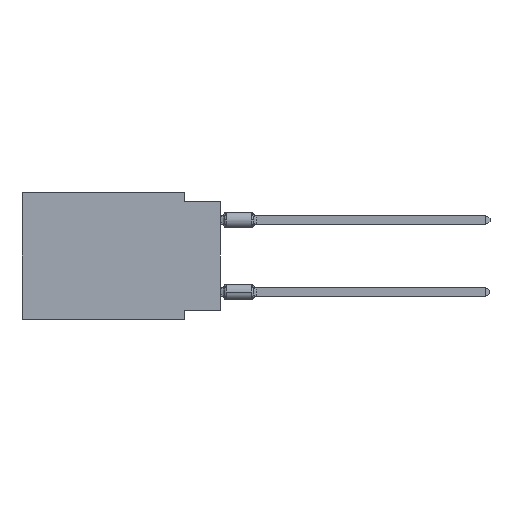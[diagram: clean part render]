
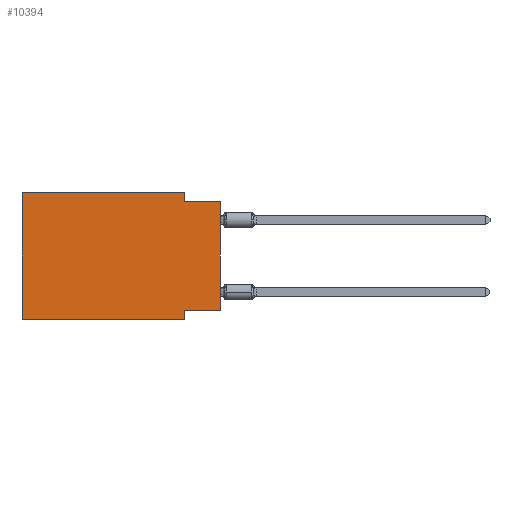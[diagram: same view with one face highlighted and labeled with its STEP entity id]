
A CAD part, left-side view. The second image highlights one B-rep face of the part: STEP entity #10394.
In plain terms, the highlighted planar face has unit normal (-1, 0, 0).
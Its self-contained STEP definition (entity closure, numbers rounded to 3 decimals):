
#94 = EDGE_CURVE ( 'NONE', #20671, #5202, #18886, .T. ) ;
#200 = LINE ( 'NONE', #1727, #14574 ) ;
#619 = CARTESIAN_POINT ( 'NONE',  ( 0., 13.97, -8.89 ) ) ;
#1194 = CARTESIAN_POINT ( 'NONE',  ( 0., 0., -0.635 ) ) ;
#1363 = ORIENTED_EDGE ( 'NONE', *, *, #13516, .F. ) ;
#1425 = PLANE ( 'NONE',  #19031 ) ;
#1727 = CARTESIAN_POINT ( 'NONE',  ( 0., 13.97, 0. ) ) ;
#1982 = EDGE_CURVE ( 'NONE', #8667, #16884, #11767, .T. ) ;
#2257 = CARTESIAN_POINT ( 'NONE',  ( 0., 2.54, -8.89 ) ) ;
#2622 = DIRECTION ( 'NONE',  ( 0., 0., 1. ) ) ;
#2673 = CARTESIAN_POINT ( 'NONE',  ( 0., 13.97, -8.89 ) ) ;
#2741 = EDGE_CURVE ( 'NONE', #5413, #16008, #200, .T. ) ;
#3243 = VERTEX_POINT ( 'NONE', #19959 ) ;
#3809 = VECTOR ( 'NONE', #13233, 1000. ) ;
#4658 = LINE ( 'NONE', #11383, #3809 ) ;
#4990 = VECTOR ( 'NONE', #8406, 1000. ) ;
#5202 = VERTEX_POINT ( 'NONE', #10467 ) ;
#5413 = VERTEX_POINT ( 'NONE', #13486 ) ;
#5815 = CARTESIAN_POINT ( 'NONE',  ( 0., 2.54, -0.635 ) ) ;
#6433 = FACE_OUTER_BOUND ( 'NONE', #13470, .T. ) ;
#6672 = DIRECTION ( 'NONE',  ( 0., 0., 1. ) ) ;
#6986 = LINE ( 'NONE', #8720, #14095 ) ;
#7366 = LINE ( 'NONE', #2257, #20247 ) ;
#7797 = CARTESIAN_POINT ( 'NONE',  ( 0., 2.54, 0. ) ) ;
#8099 = EDGE_CURVE ( 'NONE', #17785, #5202, #7366, .T. ) ;
#8141 = ORIENTED_EDGE ( 'NONE', *, *, #1982, .F. ) ;
#8174 = CARTESIAN_POINT ( 'NONE',  ( 0., 13.97, 0. ) ) ;
#8406 = DIRECTION ( 'NONE',  ( 0., -1., 0. ) ) ;
#8667 = VERTEX_POINT ( 'NONE', #5815 ) ;
#8720 = CARTESIAN_POINT ( 'NONE',  ( 0., 13.97, 0. ) ) ;
#8890 = DIRECTION ( 'NONE',  ( 0., 0., -1. ) ) ;
#9154 = ORIENTED_EDGE ( 'NONE', *, *, #8099, .F. ) ;
#9872 = VECTOR ( 'NONE', #15919, 1000. ) ;
#9995 = ORIENTED_EDGE ( 'NONE', *, *, #2741, .F. ) ;
#10394 = ADVANCED_FACE ( 'NONE', ( #6433 ), #1425, .F. ) ;
#10467 = CARTESIAN_POINT ( 'NONE',  ( 0., 2.54, -8.89 ) ) ;
#11089 = CARTESIAN_POINT ( 'NONE',  ( 0., 0., 0. ) ) ;
#11383 = CARTESIAN_POINT ( 'NONE',  ( 0., 0., -8.255 ) ) ;
#11475 = ORIENTED_EDGE ( 'NONE', *, *, #18282, .T. ) ;
#11767 = LINE ( 'NONE', #13396, #4990 ) ;
#13233 = DIRECTION ( 'NONE',  ( 0., 1., 0. ) ) ;
#13396 = CARTESIAN_POINT ( 'NONE',  ( 0., 0., -0.635 ) ) ;
#13421 = CARTESIAN_POINT ( 'NONE',  ( 0., 2.54, -8.255 ) ) ;
#13470 = EDGE_LOOP ( 'NONE', ( #11475, #8141, #1363, #9995, #17863, #18064, #9154, #17103 ) ) ;
#13486 = CARTESIAN_POINT ( 'NONE',  ( 0., 13.97, 0. ) ) ;
#13516 = EDGE_CURVE ( 'NONE', #16008, #8667, #16564, .T. ) ;
#14095 = VECTOR ( 'NONE', #6672, 1000. ) ;
#14574 = VECTOR ( 'NONE', #14974, 1000. ) ;
#14974 = DIRECTION ( 'NONE',  ( 0., -1., 0. ) ) ;
#15919 = DIRECTION ( 'NONE',  ( 0., -1., 0. ) ) ;
#16008 = VERTEX_POINT ( 'NONE', #7797 ) ;
#16564 = LINE ( 'NONE', #18526, #19294 ) ;
#16739 = DIRECTION ( 'NONE',  ( 1., 0., 0. ) ) ;
#16884 = VERTEX_POINT ( 'NONE', #1194 ) ;
#17103 = ORIENTED_EDGE ( 'NONE', *, *, #20350, .F. ) ;
#17785 = VERTEX_POINT ( 'NONE', #13421 ) ;
#17863 = ORIENTED_EDGE ( 'NONE', *, *, #21382, .F. ) ;
#18064 = ORIENTED_EDGE ( 'NONE', *, *, #94, .T. ) ;
#18282 = EDGE_CURVE ( 'NONE', #3243, #16884, #21197, .T. ) ;
#18285 = DIRECTION ( 'NONE',  ( 0., 0., -1. ) ) ;
#18526 = CARTESIAN_POINT ( 'NONE',  ( 0., 2.54, 0. ) ) ;
#18886 = LINE ( 'NONE', #2673, #9872 ) ;
#19031 = AXIS2_PLACEMENT_3D ( 'NONE', #8174, #16739, #18285 ) ;
#19294 = VECTOR ( 'NONE', #20254, 1000. ) ;
#19706 = VECTOR ( 'NONE', #2622, 1000. ) ;
#19959 = CARTESIAN_POINT ( 'NONE',  ( 0., 0., -8.255 ) ) ;
#20247 = VECTOR ( 'NONE', #8890, 1000. ) ;
#20254 = DIRECTION ( 'NONE',  ( 0., 0., -1. ) ) ;
#20350 = EDGE_CURVE ( 'NONE', #3243, #17785, #4658, .T. ) ;
#20671 = VERTEX_POINT ( 'NONE', #619 ) ;
#21197 = LINE ( 'NONE', #11089, #19706 ) ;
#21382 = EDGE_CURVE ( 'NONE', #20671, #5413, #6986, .T. ) ;
